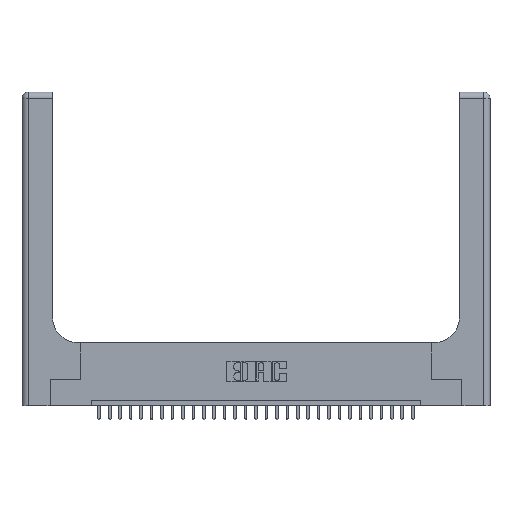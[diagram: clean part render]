
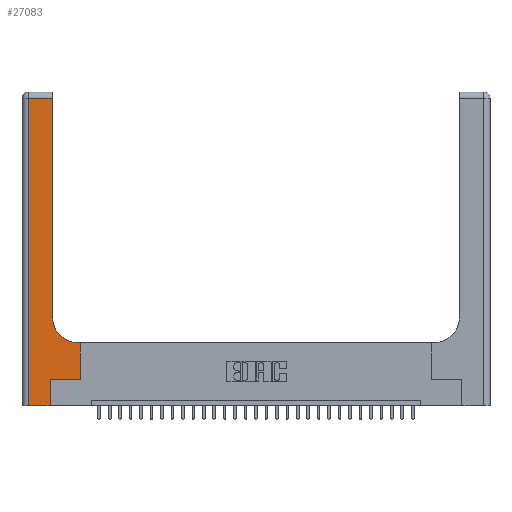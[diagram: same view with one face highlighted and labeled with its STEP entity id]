
A CAD part, top view. The second image highlights one B-rep face of the part: STEP entity #27083.
In plain terms, the highlighted planar face has unit normal (0, 0, 1).
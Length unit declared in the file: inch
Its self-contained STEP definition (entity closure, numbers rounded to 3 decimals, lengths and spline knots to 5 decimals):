
#1420 = EDGE_CURVE ( 'NONE', #20484, #7450, #14010, .T. ) ;
#2312 = VERTEX_POINT ( 'NONE', #3630 ) ;
#2407 = CIRCLE ( 'NONE', #13991, 0.25 ) ;
#2463 = EDGE_CURVE ( 'NONE', #15595, #13313, #13383, .T. ) ;
#2747 = ORIENTED_EDGE ( 'NONE', *, *, #10298, .T. ) ;
#3630 = CARTESIAN_POINT ( 'NONE',  ( 0.06, 0., 0.37 ) ) ;
#4628 = DIRECTION ( 'NONE',  ( -1., 0., 0. ) ) ;
#4813 = CARTESIAN_POINT ( 'NONE',  ( 0.2915, 0.6, 0.37 ) ) ;
#4970 = EDGE_CURVE ( 'NONE', #13312, #20484, #2407, .T. ) ;
#5785 = FACE_OUTER_BOUND ( 'NONE', #23830, .T. ) ;
#6550 = CARTESIAN_POINT ( 'NONE',  ( 0.269, 0.25, 0.37 ) ) ;
#7198 = LINE ( 'NONE', #28544, #15897 ) ;
#7450 = VERTEX_POINT ( 'NONE', #14626 ) ;
#7500 = CARTESIAN_POINT ( 'NONE',  ( 0.5415, 0.6, 0.37 ) ) ;
#8340 = CARTESIAN_POINT ( 'NONE',  ( 0.269, 0., 0.37 ) ) ;
#10298 = EDGE_CURVE ( 'NONE', #13037, #2312, #24727, .T. ) ;
#10459 = DIRECTION ( 'NONE',  ( 1., 0., 0. ) ) ;
#10503 = EDGE_CURVE ( 'NONE', #26867, #15595, #21396, .T. ) ;
#10680 = ORIENTED_EDGE ( 'NONE', *, *, #24123, .T. ) ;
#10818 = CARTESIAN_POINT ( 'NONE',  ( 0., 3., 0.37 ) ) ;
#11012 = DIRECTION ( 'NONE',  ( -1., 0., 0. ) ) ;
#11081 = ORIENTED_EDGE ( 'NONE', *, *, #22073, .T. ) ;
#11410 = CARTESIAN_POINT ( 'NONE',  ( 0.06, 3., 0.37 ) ) ;
#11985 = VECTOR ( 'NONE', #29358, 39.37008 ) ;
#12734 = CARTESIAN_POINT ( 'NONE',  ( 0.2915, 3., 0.37 ) ) ;
#13037 = VERTEX_POINT ( 'NONE', #18170 ) ;
#13312 = VERTEX_POINT ( 'NONE', #7500 ) ;
#13313 = VERTEX_POINT ( 'NONE', #13792 ) ;
#13359 = PLANE ( 'NONE',  #14771 ) ;
#13383 = LINE ( 'NONE', #16830, #23165 ) ;
#13792 = CARTESIAN_POINT ( 'NONE',  ( 0.5585, 0.6, 0.37 ) ) ;
#13991 = AXIS2_PLACEMENT_3D ( 'NONE', #22475, #29144, #17565 ) ;
#14010 = LINE ( 'NONE', #12734, #28147 ) ;
#14626 = CARTESIAN_POINT ( 'NONE',  ( 0.2915, 2.94, 0.37 ) ) ;
#14771 = AXIS2_PLACEMENT_3D ( 'NONE', #10818, #20213, #11012 ) ;
#15031 = EDGE_CURVE ( 'NONE', #16247, #26867, #22213, .T. ) ;
#15060 = CARTESIAN_POINT ( 'NONE',  ( 0.2915, 0.85, 0.37 ) ) ;
#15595 = VERTEX_POINT ( 'NONE', #21828 ) ;
#15897 = VECTOR ( 'NONE', #26966, 39.37008 ) ;
#16042 = LINE ( 'NONE', #24384, #27022 ) ;
#16247 = VERTEX_POINT ( 'NONE', #21540 ) ;
#16830 = CARTESIAN_POINT ( 'NONE',  ( 0.5585, 0.25, 0.37 ) ) ;
#17565 = DIRECTION ( 'NONE',  ( 1., 0., 0. ) ) ;
#18170 = CARTESIAN_POINT ( 'NONE',  ( 0.06, 2.94, 0.37 ) ) ;
#18353 = VECTOR ( 'NONE', #4628, 39.37008 ) ;
#19747 = ORIENTED_EDGE ( 'NONE', *, *, #15031, .T. ) ;
#20213 = DIRECTION ( 'NONE',  ( 0., 0., -1. ) ) ;
#20484 = VERTEX_POINT ( 'NONE', #15060 ) ;
#21025 = EDGE_CURVE ( 'NONE', #7450, #13037, #7198, .T. ) ;
#21262 = LINE ( 'NONE', #4813, #18353 ) ;
#21396 = LINE ( 'NONE', #6550, #11985 ) ;
#21540 = CARTESIAN_POINT ( 'NONE',  ( 0.269, 0., 0.37 ) ) ;
#21828 = CARTESIAN_POINT ( 'NONE',  ( 0.5585, 0.25, 0.37 ) ) ;
#21874 = ORIENTED_EDGE ( 'NONE', *, *, #21025, .T. ) ;
#22073 = EDGE_CURVE ( 'NONE', #13313, #13312, #21262, .T. ) ;
#22213 = LINE ( 'NONE', #8340, #28717 ) ;
#22475 = CARTESIAN_POINT ( 'NONE',  ( 0.5415, 0.85, 0.37 ) ) ;
#23165 = VECTOR ( 'NONE', #24367, 39.37008 ) ;
#23830 = EDGE_LOOP ( 'NONE', ( #25986, #21874, #2747, #10680, #19747, #25279, #29046, #11081, #26947 ) ) ;
#23889 = DIRECTION ( 'NONE',  ( 0., 1., 0. ) ) ;
#24123 = EDGE_CURVE ( 'NONE', #2312, #16247, #16042, .T. ) ;
#24367 = DIRECTION ( 'NONE',  ( 0., 1., 0. ) ) ;
#24384 = CARTESIAN_POINT ( 'NONE',  ( 0., 0., 0.37 ) ) ;
#24727 = LINE ( 'NONE', #11410, #29074 ) ;
#25279 = ORIENTED_EDGE ( 'NONE', *, *, #10503, .T. ) ;
#25459 = CARTESIAN_POINT ( 'NONE',  ( 0.269, 0.25, 0.37 ) ) ;
#25986 = ORIENTED_EDGE ( 'NONE', *, *, #1420, .T. ) ;
#26757 = DIRECTION ( 'NONE',  ( 0., 1., 0. ) ) ;
#26867 = VERTEX_POINT ( 'NONE', #25459 ) ;
#26947 = ORIENTED_EDGE ( 'NONE', *, *, #4970, .T. ) ;
#26966 = DIRECTION ( 'NONE',  ( -1., 0., 0. ) ) ;
#27022 = VECTOR ( 'NONE', #10459, 39.37008 ) ;
#27083 = ADVANCED_FACE ( 'NONE', ( #5785 ), #13359, .F. ) ;
#27952 = DIRECTION ( 'NONE',  ( 0., -1., 0. ) ) ;
#28147 = VECTOR ( 'NONE', #23889, 39.37008 ) ;
#28544 = CARTESIAN_POINT ( 'NONE',  ( 0., 2.94, 0.37 ) ) ;
#28717 = VECTOR ( 'NONE', #26757, 39.37008 ) ;
#29046 = ORIENTED_EDGE ( 'NONE', *, *, #2463, .T. ) ;
#29074 = VECTOR ( 'NONE', #27952, 39.37008 ) ;
#29144 = DIRECTION ( 'NONE',  ( 0., 0., -1. ) ) ;
#29358 = DIRECTION ( 'NONE',  ( 1., 0., 0. ) ) ;
